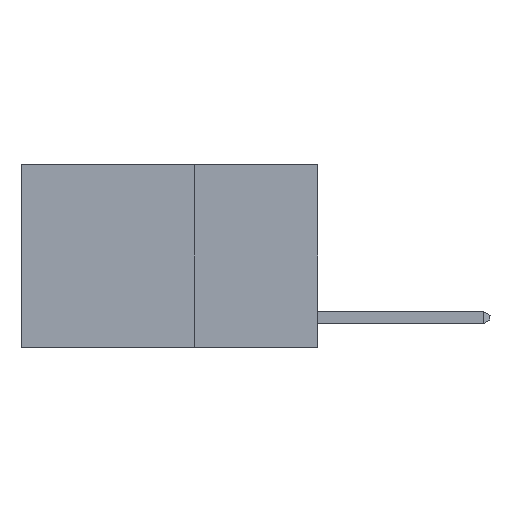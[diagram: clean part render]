
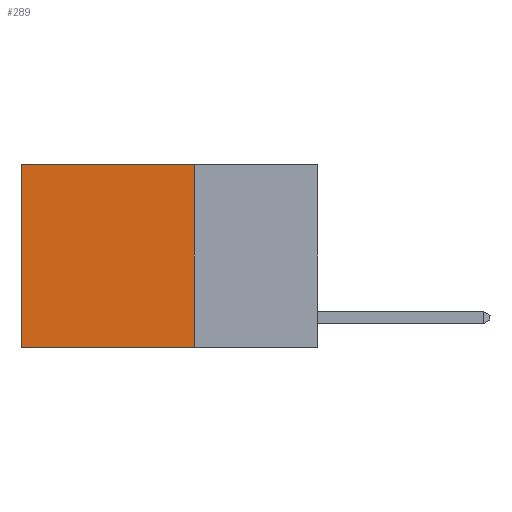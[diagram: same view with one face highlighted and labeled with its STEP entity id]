
A CAD part, left-side view. The second image highlights one B-rep face of the part: STEP entity #289.
In plain terms, the highlighted planar face has unit normal (-1, 0, 0).
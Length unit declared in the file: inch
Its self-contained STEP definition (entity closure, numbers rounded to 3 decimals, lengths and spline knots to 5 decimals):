
#289 = ADVANCED_FACE ( 'NONE', ( #6078 ), #20968, .F. ) ;
#377 = ORIENTED_EDGE ( 'NONE', *, *, #20628, .T. ) ;
#1110 = LINE ( 'NONE', #11688, #5022 ) ;
#1147 = DIRECTION ( 'NONE',  ( 1., 0., 0. ) ) ;
#1740 = VERTEX_POINT ( 'NONE', #11525 ) ;
#1893 = EDGE_LOOP ( 'NONE', ( #18205, #2140, #16489, #377 ) ) ;
#2140 = ORIENTED_EDGE ( 'NONE', *, *, #19828, .F. ) ;
#2800 = VERTEX_POINT ( 'NONE', #11646 ) ;
#2945 = DIRECTION ( 'NONE',  ( 0., 1., 0. ) ) ;
#3795 = LINE ( 'NONE', #20292, #17498 ) ;
#5022 = VECTOR ( 'NONE', #13366, 39.37008 ) ;
#6078 = FACE_OUTER_BOUND ( 'NONE', #1893, .T. ) ;
#6428 = EDGE_CURVE ( 'NONE', #2800, #8015, #14308, .T. ) ;
#8015 = VERTEX_POINT ( 'NONE', #20590 ) ;
#8757 = DIRECTION ( 'NONE',  ( 0., 1., 0. ) ) ;
#9420 = CARTESIAN_POINT ( 'NONE',  ( 0.2625, 0.25, 0. ) ) ;
#9543 = DIRECTION ( 'NONE',  ( 0., 0., -1. ) ) ;
#11525 = CARTESIAN_POINT ( 'NONE',  ( 0.2625, 0.6, 0. ) ) ;
#11576 = LINE ( 'NONE', #12840, #20363 ) ;
#11646 = CARTESIAN_POINT ( 'NONE',  ( 0.2625, 0.25, 0. ) ) ;
#11688 = CARTESIAN_POINT ( 'NONE',  ( 0.2625, 0.6, 0. ) ) ;
#12732 = DIRECTION ( 'NONE',  ( 0., 0., -1. ) ) ;
#12840 = CARTESIAN_POINT ( 'NONE',  ( 0.2625, 0.25, -0.37 ) ) ;
#13277 = AXIS2_PLACEMENT_3D ( 'NONE', #9420, #1147, #12732 ) ;
#13366 = DIRECTION ( 'NONE',  ( 0., 0., -1. ) ) ;
#14308 = LINE ( 'NONE', #19442, #14824 ) ;
#14824 = VECTOR ( 'NONE', #9543, 39.37008 ) ;
#16192 = EDGE_CURVE ( 'NONE', #1740, #16673, #1110, .T. ) ;
#16489 = ORIENTED_EDGE ( 'NONE', *, *, #6428, .F. ) ;
#16673 = VERTEX_POINT ( 'NONE', #19694 ) ;
#17498 = VECTOR ( 'NONE', #8757, 39.37008 ) ;
#18205 = ORIENTED_EDGE ( 'NONE', *, *, #16192, .T. ) ;
#19442 = CARTESIAN_POINT ( 'NONE',  ( 0.2625, 0.25, 0. ) ) ;
#19694 = CARTESIAN_POINT ( 'NONE',  ( 0.2625, 0.6, -0.37 ) ) ;
#19828 = EDGE_CURVE ( 'NONE', #8015, #16673, #11576, .T. ) ;
#20292 = CARTESIAN_POINT ( 'NONE',  ( 0.2625, 0.25, 0. ) ) ;
#20363 = VECTOR ( 'NONE', #2945, 39.37008 ) ;
#20590 = CARTESIAN_POINT ( 'NONE',  ( 0.2625, 0.25, -0.37 ) ) ;
#20628 = EDGE_CURVE ( 'NONE', #2800, #1740, #3795, .T. ) ;
#20968 = PLANE ( 'NONE',  #13277 ) ;
